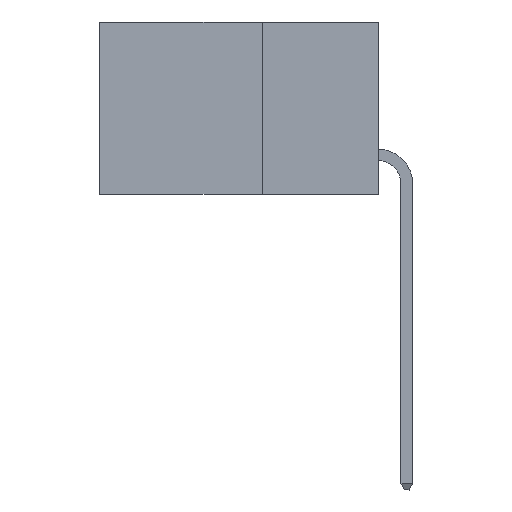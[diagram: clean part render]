
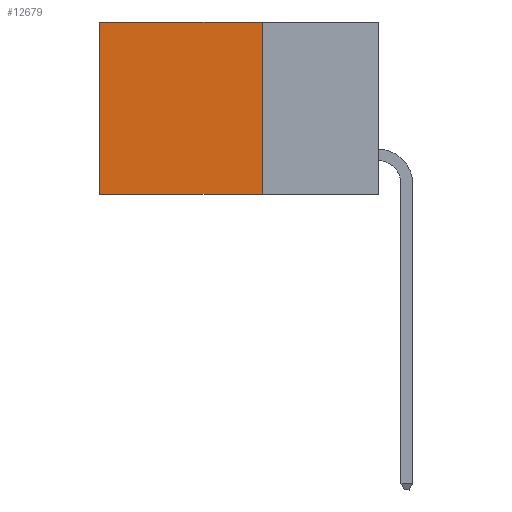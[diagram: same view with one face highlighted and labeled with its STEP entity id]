
A CAD part, left-side view. The second image highlights one B-rep face of the part: STEP entity #12679.
In plain terms, the highlighted planar face has unit normal (-1, 0, 0).
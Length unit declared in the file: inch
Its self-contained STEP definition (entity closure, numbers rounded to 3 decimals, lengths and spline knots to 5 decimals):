
#65 = CARTESIAN_POINT ( 'NONE',  ( 0.2615, 0.25, -0.37 ) ) ;
#298 = EDGE_CURVE ( 'NONE', #8130, #9352, #10191, .T. ) ;
#400 = DIRECTION ( 'NONE',  ( 0., 0., -1. ) ) ;
#975 = CARTESIAN_POINT ( 'NONE',  ( 0.2615, 0.6, 0. ) ) ;
#1619 = ORIENTED_EDGE ( 'NONE', *, *, #10939, .T. ) ;
#2699 = LINE ( 'NONE', #9151, #13519 ) ;
#2824 = CARTESIAN_POINT ( 'NONE',  ( 0.2615, 0.25, -0.37 ) ) ;
#3293 = LINE ( 'NONE', #6218, #9083 ) ;
#3538 = CARTESIAN_POINT ( 'NONE',  ( 0.2615, 0.6, -0.37 ) ) ;
#4180 = EDGE_CURVE ( 'NONE', #9352, #11416, #2699, .T. ) ;
#4327 = DIRECTION ( 'NONE',  ( 1., 0., 0. ) ) ;
#4437 = VERTEX_POINT ( 'NONE', #975 ) ;
#5037 = CARTESIAN_POINT ( 'NONE',  ( 0.2615, 0.25, 0. ) ) ;
#5260 = DIRECTION ( 'NONE',  ( 0., 1., 0. ) ) ;
#6045 = DIRECTION ( 'NONE',  ( 0., 1., 0. ) ) ;
#6145 = CARTESIAN_POINT ( 'NONE',  ( 0.2615, 0.6, -0.37 ) ) ;
#6218 = CARTESIAN_POINT ( 'NONE',  ( 0.2615, 0.25, 0. ) ) ;
#6219 = AXIS2_PLACEMENT_3D ( 'NONE', #65, #4327, #8545 ) ;
#6932 = ORIENTED_EDGE ( 'NONE', *, *, #4180, .F. ) ;
#6988 = VECTOR ( 'NONE', #400, 39.37008 ) ;
#7956 = ORIENTED_EDGE ( 'NONE', *, *, #12891, .T. ) ;
#8130 = VERTEX_POINT ( 'NONE', #5037 ) ;
#8545 = DIRECTION ( 'NONE',  ( 0., 0., -1. ) ) ;
#8665 = EDGE_LOOP ( 'NONE', ( #1619, #6932, #12153, #7956 ) ) ;
#8950 = CARTESIAN_POINT ( 'NONE',  ( 0.2615, 0.25, -0.37 ) ) ;
#9083 = VECTOR ( 'NONE', #5260, 39.37008 ) ;
#9151 = CARTESIAN_POINT ( 'NONE',  ( 0.2615, 0.25, -0.37 ) ) ;
#9352 = VERTEX_POINT ( 'NONE', #8950 ) ;
#9947 = VECTOR ( 'NONE', #13099, 39.37008 ) ;
#10191 = LINE ( 'NONE', #2824, #6988 ) ;
#10609 = PLANE ( 'NONE',  #6219 ) ;
#10939 = EDGE_CURVE ( 'NONE', #4437, #11416, #13018, .T. ) ;
#11416 = VERTEX_POINT ( 'NONE', #6145 ) ;
#12153 = ORIENTED_EDGE ( 'NONE', *, *, #298, .F. ) ;
#12679 = ADVANCED_FACE ( 'NONE', ( #13022 ), #10609, .F. ) ;
#12891 = EDGE_CURVE ( 'NONE', #8130, #4437, #3293, .T. ) ;
#13018 = LINE ( 'NONE', #3538, #9947 ) ;
#13022 = FACE_OUTER_BOUND ( 'NONE', #8665, .T. ) ;
#13099 = DIRECTION ( 'NONE',  ( 0., 0., -1. ) ) ;
#13519 = VECTOR ( 'NONE', #6045, 39.37008 ) ;
